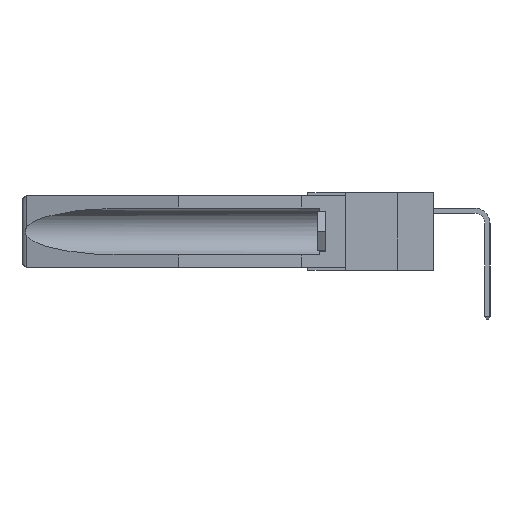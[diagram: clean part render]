
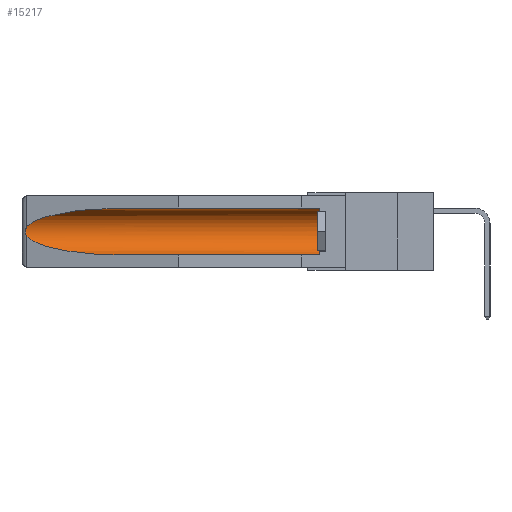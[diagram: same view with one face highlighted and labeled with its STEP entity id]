
A CAD part, left-side view. The second image highlights one B-rep face of the part: STEP entity #15217.
In plain terms, the highlighted cylindrical face has radius 2.857 mm (diameter 5.715 mm), a partial arc.
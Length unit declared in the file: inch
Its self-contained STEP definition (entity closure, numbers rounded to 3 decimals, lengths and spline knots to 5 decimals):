
#12 = DIRECTION ( 'NONE',  ( 0., 0., 1. ) ) ;
#43 = CARTESIAN_POINT ( 'NONE',  ( 0.26597, 1.5296, -0.19026 ) ) ;
#429 =( BOUNDED_CURVE ( )  B_SPLINE_CURVE ( 3, ( #1720, #8634, #15309, #14047 ),
 .UNSPECIFIED., .F., .F. ) 
 B_SPLINE_CURVE_WITH_KNOTS ( ( 4, 4 ),
 ( 0.1948, 1.5708 ),
 .UNSPECIFIED. ) 
 CURVE ( )  GEOMETRIC_REPRESENTATION_ITEM ( )  RATIONAL_B_SPLINE_CURVE ( ( 1., 0.848, 0.848, 1. ) ) 
 REPRESENTATION_ITEM ( '' )  );
#481 = CIRCLE ( 'NONE', #1904, 0.1125 ) ;
#643 = DIRECTION ( 'NONE',  ( 0., 1., 0. ) ) ;
#1234 = CARTESIAN_POINT ( 'NONE',  ( 0.2673, 1.5327, -0.16383 ) ) ;
#1320 = CARTESIAN_POINT ( 'NONE',  ( 0.155, 0.126, -0.1715 ) ) ;
#1341 = FACE_OUTER_BOUND ( 'NONE', #15442, .T. ) ;
#1418 = DIRECTION ( 'NONE',  ( 0., 1., 0. ) ) ;
#1720 = CARTESIAN_POINT ( 'NONE',  ( 0.26537, 1.52718, -0.19328 ) ) ;
#1904 = AXIS2_PLACEMENT_3D ( 'NONE', #1320, #8046, #12 ) ;
#2516 = LINE ( 'NONE', #16669, #12773 ) ;
#2592 = CARTESIAN_POINT ( 'NONE',  ( 0.2675, 1.53308, -0.16763 ) ) ;
#2802 = CYLINDRICAL_SURFACE ( 'NONE', #5858, 0.1125 ) ;
#4899 = CARTESIAN_POINT ( 'NONE',  ( 0.155, 1.07973, -0.284 ) ) ;
#5297 = CARTESIAN_POINT ( 'NONE',  ( 0.26537, 1.52718, -0.19328 ) ) ;
#5858 = AXIS2_PLACEMENT_3D ( 'NONE', #9958, #9841, #11414 ) ;
#6012 = VERTEX_POINT ( 'NONE', #7802 ) ;
#6171 = CARTESIAN_POINT ( 'NONE',  ( 0.26537, 1.52718, -0.14972 ) ) ;
#6661 = CARTESIAN_POINT ( 'NONE',  ( 0.26655, 1.53094, -0.18657 ) ) ;
#6751 = VERTEX_POINT ( 'NONE', #16801 ) ;
#6762 = VERTEX_POINT ( 'NONE', #16732 ) ;
#6927 = ORIENTED_EDGE ( 'NONE', *, *, #12200, .T. ) ;
#7588 = VERTEX_POINT ( 'NONE', #9124 ) ;
#7802 = CARTESIAN_POINT ( 'NONE',  ( 0.155, 0.126, -0.284 ) ) ;
#7965 = CARTESIAN_POINT ( 'NONE',  ( 0.2675, 1.53308, -0.17534 ) ) ;
#8046 = DIRECTION ( 'NONE',  ( 0., -1., 0. ) ) ;
#8084 = CARTESIAN_POINT ( 'NONE',  ( 0.2673, 1.53269, -0.17917 ) ) ;
#8634 = CARTESIAN_POINT ( 'NONE',  ( 0.25451, 1.48313, -0.24835 ) ) ;
#9124 = CARTESIAN_POINT ( 'NONE',  ( 0.26537, 1.52718, -0.14972 ) ) ;
#9566 = EDGE_CURVE ( 'NONE', #6012, #6751, #481, .T. ) ;
#9612 = VERTEX_POINT ( 'NONE', #11874 ) ;
#9841 = DIRECTION ( 'NONE',  ( 0., 1., 0. ) ) ;
#9958 = CARTESIAN_POINT ( 'NONE',  ( 0.155, -0.30754, -0.1715 ) ) ;
#10123 = CARTESIAN_POINT ( 'NONE',  ( 0.25451, 1.48313, -0.09465 ) ) ;
#10280 = VECTOR ( 'NONE', #1418, 39.37008 ) ;
#11068 = ORIENTED_EDGE ( 'NONE', *, *, #11318, .T. ) ;
#11318 = EDGE_CURVE ( 'NONE', #6751, #9612, #12370, .T. ) ;
#11414 = DIRECTION ( 'NONE',  ( 0., 0., 1. ) ) ;
#11489 = EDGE_CURVE ( 'NONE', #9612, #7588, #17036, .T. ) ;
#11772 = EDGE_CURVE ( 'NONE', #6762, #16355, #429, .T. ) ;
#11874 = CARTESIAN_POINT ( 'NONE',  ( 0.155, 1.07973, -0.059 ) ) ;
#11932 = ORIENTED_EDGE ( 'NONE', *, *, #11772, .T. ) ;
#11988 = ORIENTED_EDGE ( 'NONE', *, *, #11489, .T. ) ;
#12200 = EDGE_CURVE ( 'NONE', #7588, #6762, #12369, .T. ) ;
#12370 = LINE ( 'NONE', #17300, #10280 ) ;
#12369 = B_SPLINE_CURVE_WITH_KNOTS ( 'NONE', 3,
 ( #16080, #17283, #13226, #1234, #2592, #7965, #8084, #6661, #43, #5297 ),
 .UNSPECIFIED., .F., .F.,
 ( 4, 2, 2, 2, 4 ),
 ( 0., 0.00029, 0.00058, 0.00087, 0.00117 ),
 .UNSPECIFIED. ) ;
#12773 = VECTOR ( 'NONE', #643, 39.37008 ) ;
#13226 = CARTESIAN_POINT ( 'NONE',  ( 0.26654, 1.53092, -0.15636 ) ) ;
#13776 = CARTESIAN_POINT ( 'NONE',  ( 0.21114, 1.30732, -0.059 ) ) ;
#13946 = CARTESIAN_POINT ( 'NONE',  ( 0.155, 1.07973, -0.059 ) ) ;
#14047 = CARTESIAN_POINT ( 'NONE',  ( 0.155, 1.07973, -0.284 ) ) ;
#15217 = ADVANCED_FACE ( 'NONE', ( #1341 ), #2802, .F. ) ;
#15309 = CARTESIAN_POINT ( 'NONE',  ( 0.21114, 1.30732, -0.284 ) ) ;
#15442 = EDGE_LOOP ( 'NONE', ( #11988, #6927, #11932, #16190, #16288, #11068 ) ) ;
#16080 = CARTESIAN_POINT ( 'NONE',  ( 0.26537, 1.52718, -0.14972 ) ) ;
#16190 = ORIENTED_EDGE ( 'NONE', *, *, #16846, .F. ) ;
#16288 = ORIENTED_EDGE ( 'NONE', *, *, #9566, .T. ) ;
#16355 = VERTEX_POINT ( 'NONE', #4899 ) ;
#16669 = CARTESIAN_POINT ( 'NONE',  ( 0.155, -0.30754, -0.284 ) ) ;
#16732 = CARTESIAN_POINT ( 'NONE',  ( 0.26537, 1.52718, -0.19328 ) ) ;
#16801 = CARTESIAN_POINT ( 'NONE',  ( 0.155, 0.126, -0.059 ) ) ;
#16846 = EDGE_CURVE ( 'NONE', #6012, #16355, #2516, .T. ) ;
#17036 =( BOUNDED_CURVE ( )  B_SPLINE_CURVE ( 3, ( #13946, #13776, #10123, #6171 ),
 .UNSPECIFIED., .F., .F. ) 
 B_SPLINE_CURVE_WITH_KNOTS ( ( 4, 4 ),
 ( 4.71239, 6.08839 ),
 .UNSPECIFIED. ) 
 CURVE ( )  GEOMETRIC_REPRESENTATION_ITEM ( )  RATIONAL_B_SPLINE_CURVE ( ( 1., 0.848, 0.848, 1. ) ) 
 REPRESENTATION_ITEM ( '' )  );
#17283 = CARTESIAN_POINT ( 'NONE',  ( 0.26597, 1.52961, -0.15275 ) ) ;
#17300 = CARTESIAN_POINT ( 'NONE',  ( 0.155, -0.30754, -0.059 ) ) ;
